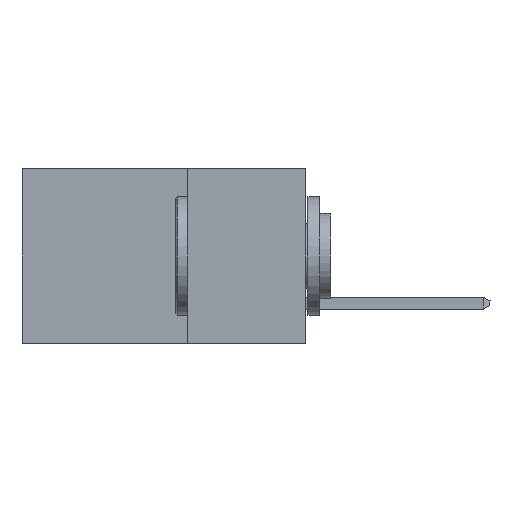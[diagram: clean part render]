
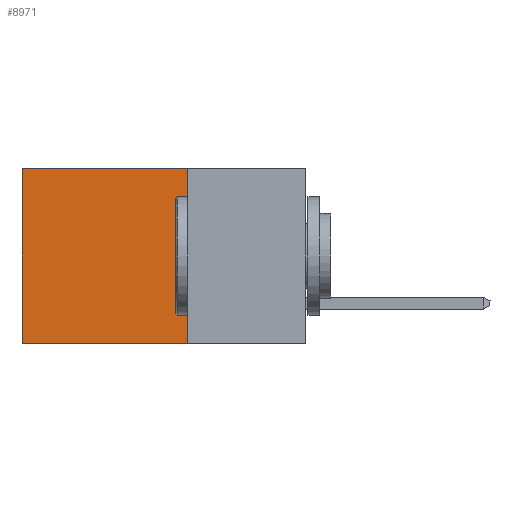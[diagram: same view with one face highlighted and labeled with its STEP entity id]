
A CAD part, left-side view. The second image highlights one B-rep face of the part: STEP entity #8971.
In plain terms, the highlighted planar face has unit normal (-1, 0, 0).
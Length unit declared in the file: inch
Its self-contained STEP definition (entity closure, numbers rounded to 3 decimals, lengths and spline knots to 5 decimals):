
#132 = CARTESIAN_POINT ( 'NONE',  ( 0.298, 0.25, 0. ) ) ;
#196 = CARTESIAN_POINT ( 'NONE',  ( 0.298, 0.25, -0.37 ) ) ;
#1456 = CARTESIAN_POINT ( 'NONE',  ( 0.298, 0.6, 0. ) ) ;
#1992 = DIRECTION ( 'NONE',  ( 0., 0., -1. ) ) ;
#4227 = PLANE ( 'NONE',  #6698 ) ;
#4320 = VERTEX_POINT ( 'NONE', #22905 ) ;
#4665 = EDGE_CURVE ( 'NONE', #20637, #4320, #28956, .T. ) ;
#4694 = DIRECTION ( 'NONE',  ( 0., 1., 0. ) ) ;
#5287 = LINE ( 'NONE', #23022, #11128 ) ;
#5776 = VECTOR ( 'NONE', #24314, 39.37008 ) ;
#6698 = AXIS2_PLACEMENT_3D ( 'NONE', #13295, #22391, #1992 ) ;
#7267 = VECTOR ( 'NONE', #23680, 39.37008 ) ;
#8541 = CARTESIAN_POINT ( 'NONE',  ( 0.298, 0.6, 0. ) ) ;
#8971 = ADVANCED_FACE ( 'NONE', ( #24628 ), #4227, .F. ) ;
#9165 = EDGE_CURVE ( 'NONE', #12184, #23340, #28940, .T. ) ;
#9489 = VECTOR ( 'NONE', #17617, 39.37008 ) ;
#10347 = ORIENTED_EDGE ( 'NONE', *, *, #10655, .F. ) ;
#10655 = EDGE_CURVE ( 'NONE', #23340, #4320, #15023, .T. ) ;
#11128 = VECTOR ( 'NONE', #4694, 39.37008 ) ;
#11304 = ORIENTED_EDGE ( 'NONE', *, *, #24844, .T. ) ;
#12184 = VERTEX_POINT ( 'NONE', #132 ) ;
#13295 = CARTESIAN_POINT ( 'NONE',  ( 0.298, 0.25, 0. ) ) ;
#14915 = CARTESIAN_POINT ( 'NONE',  ( 0.298, 0.25, 0. ) ) ;
#15023 = LINE ( 'NONE', #25781, #7267 ) ;
#17617 = DIRECTION ( 'NONE',  ( 0., 0., -1. ) ) ;
#20637 = VERTEX_POINT ( 'NONE', #1456 ) ;
#22391 = DIRECTION ( 'NONE',  ( 1., 0., 0. ) ) ;
#22905 = CARTESIAN_POINT ( 'NONE',  ( 0.298, 0.6, -0.37 ) ) ;
#23022 = CARTESIAN_POINT ( 'NONE',  ( 0.298, 0.25, 0. ) ) ;
#23340 = VERTEX_POINT ( 'NONE', #196 ) ;
#23680 = DIRECTION ( 'NONE',  ( 0., 1., 0. ) ) ;
#24314 = DIRECTION ( 'NONE',  ( 0., 0., -1. ) ) ;
#24628 = FACE_OUTER_BOUND ( 'NONE', #24633, .T. ) ;
#24633 = EDGE_LOOP ( 'NONE', ( #27336, #10347, #28758, #11304 ) ) ;
#24844 = EDGE_CURVE ( 'NONE', #12184, #20637, #5287, .T. ) ;
#25781 = CARTESIAN_POINT ( 'NONE',  ( 0.298, 0.25, -0.37 ) ) ;
#27336 = ORIENTED_EDGE ( 'NONE', *, *, #4665, .T. ) ;
#28758 = ORIENTED_EDGE ( 'NONE', *, *, #9165, .F. ) ;
#28940 = LINE ( 'NONE', #14915, #5776 ) ;
#28956 = LINE ( 'NONE', #8541, #9489 ) ;
